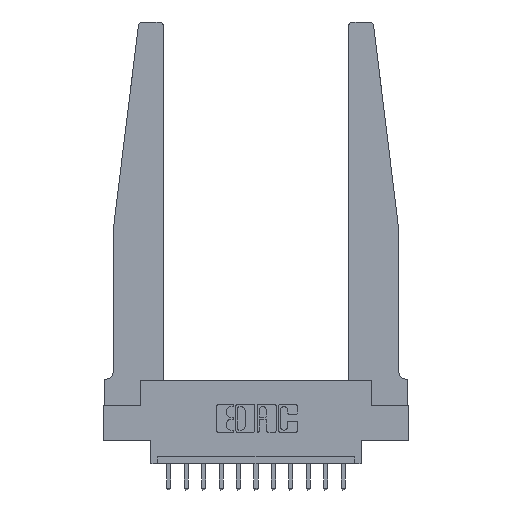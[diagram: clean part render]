
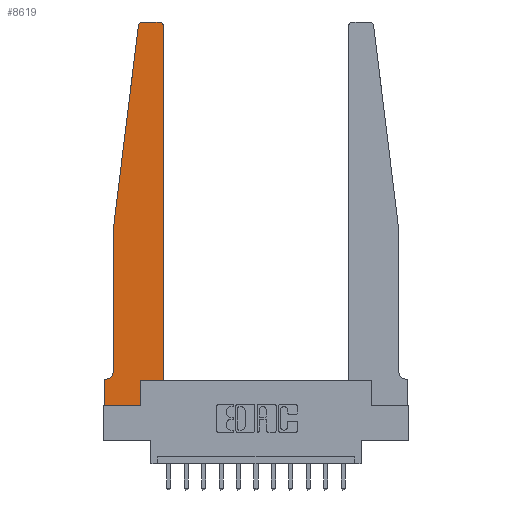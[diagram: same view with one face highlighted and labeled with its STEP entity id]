
A CAD part, top view. The second image highlights one B-rep face of the part: STEP entity #8619.
In plain terms, the highlighted planar face has unit normal (0, 0, 1).
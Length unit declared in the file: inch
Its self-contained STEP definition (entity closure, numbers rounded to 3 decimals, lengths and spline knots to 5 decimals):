
#28 = EDGE_CURVE ( 'NONE', #14382, #12071, #12122, .T. ) ;
#48 = CARTESIAN_POINT ( 'NONE',  ( 0.27653, 2.72, 0.37 ) ) ;
#54 = CARTESIAN_POINT ( 'NONE',  ( 0.27653, 2.75, 0.37 ) ) ;
#394 = CARTESIAN_POINT ( 'NONE',  ( 0.425, 0.18, 0.37 ) ) ;
#505 = LINE ( 'NONE', #9838, #10966 ) ;
#746 = EDGE_CURVE ( 'NONE', #7566, #3787, #5957, .T. ) ;
#974 = CIRCLE ( 'NONE', #13936, 0.03 ) ;
#1080 = ORIENTED_EDGE ( 'NONE', *, *, #1989, .T. ) ;
#1098 = VERTEX_POINT ( 'NONE', #54 ) ;
#1146 = EDGE_CURVE ( 'NONE', #8508, #3906, #505, .T. ) ;
#1158 = LINE ( 'NONE', #11549, #9506 ) ;
#1288 = DIRECTION ( 'NONE',  ( 0., 0., 1. ) ) ;
#1580 = CARTESIAN_POINT ( 'NONE',  ( 0., 0.1875, 0.37 ) ) ;
#1983 = CARTESIAN_POINT ( 'NONE',  ( 0., 0., 0.37 ) ) ;
#1989 = EDGE_CURVE ( 'NONE', #6457, #1098, #10658, .T. ) ;
#2303 = DIRECTION ( 'NONE',  ( 0., 0., -1. ) ) ;
#2360 = EDGE_CURVE ( 'NONE', #13261, #15558, #4961, .T. ) ;
#2396 = VECTOR ( 'NONE', #4013, 39.37008 ) ;
#2405 = DIRECTION ( 'NONE',  ( -1., 0., 0. ) ) ;
#2742 = DIRECTION ( 'NONE',  ( 0., 1., 0. ) ) ;
#2877 = EDGE_CURVE ( 'NONE', #1098, #14382, #974, .T. ) ;
#2994 = CARTESIAN_POINT ( 'NONE',  ( 0.065, 1.25, 0.37 ) ) ;
#3413 = CIRCLE ( 'NONE', #8159, 0.05 ) ;
#3787 = VERTEX_POINT ( 'NONE', #10122 ) ;
#3796 = DIRECTION ( 'NONE',  ( 1., 0., 0. ) ) ;
#3899 = CARTESIAN_POINT ( 'NONE',  ( 0., 0.1875, 0.37 ) ) ;
#3906 = VERTEX_POINT ( 'NONE', #1580 ) ;
#4013 = DIRECTION ( 'NONE',  ( -0.122, -0.992, 0. ) ) ;
#4871 = ORIENTED_EDGE ( 'NONE', *, *, #2877, .T. ) ;
#4961 = LINE ( 'NONE', #394, #12158 ) ;
#5356 = DIRECTION ( 'NONE',  ( 1., 0., 0. ) ) ;
#5385 = CARTESIAN_POINT ( 'NONE',  ( 0., 0., 0.37 ) ) ;
#5846 = CARTESIAN_POINT ( 'NONE',  ( 0.2605, 0., 0.37 ) ) ;
#5957 = LINE ( 'NONE', #9112, #7497 ) ;
#6034 = CARTESIAN_POINT ( 'NONE',  ( 0.065, 1.25, 0.37 ) ) ;
#6059 = CARTESIAN_POINT ( 'NONE',  ( 0.065, 0.2375, 0.37 ) ) ;
#6457 = VERTEX_POINT ( 'NONE', #13063 ) ;
#6497 = DIRECTION ( 'NONE',  ( 1., 0., 0. ) ) ;
#6734 = EDGE_CURVE ( 'NONE', #3787, #13261, #1158, .T. ) ;
#7161 = EDGE_CURVE ( 'NONE', #3906, #9152, #12614, .T. ) ;
#7271 = VERTEX_POINT ( 'NONE', #6059 ) ;
#7497 = VECTOR ( 'NONE', #15308, 39.37008 ) ;
#7566 = VERTEX_POINT ( 'NONE', #5846 ) ;
#7696 = ORIENTED_EDGE ( 'NONE', *, *, #6734, .T. ) ;
#7759 = ORIENTED_EDGE ( 'NONE', *, *, #1146, .T. ) ;
#7770 = DIRECTION ( 'NONE',  ( 1., 0., 0. ) ) ;
#8121 = ORIENTED_EDGE ( 'NONE', *, *, #15650, .T. ) ;
#8159 = AXIS2_PLACEMENT_3D ( 'NONE', #12286, #2303, #2405 ) ;
#8188 = CARTESIAN_POINT ( 'NONE',  ( 0.24675, 2.72367, 0.37 ) ) ;
#8312 = DIRECTION ( 'NONE',  ( 0., -1., 0. ) ) ;
#8508 = VERTEX_POINT ( 'NONE', #12459 ) ;
#8619 = ADVANCED_FACE ( 'NONE', ( #10020 ), #11304, .T. ) ;
#8872 = VECTOR ( 'NONE', #6497, 39.37008 ) ;
#9112 = CARTESIAN_POINT ( 'NONE',  ( 0.2605, 0.18, 0.37 ) ) ;
#9152 = VERTEX_POINT ( 'NONE', #14623 ) ;
#9506 = VECTOR ( 'NONE', #7770, 39.37008 ) ;
#9586 = EDGE_CURVE ( 'NONE', #15558, #6457, #14068, .T. ) ;
#9811 = DIRECTION ( 'NONE',  ( -1., 0., 0. ) ) ;
#9838 = CARTESIAN_POINT ( 'NONE',  ( 0.065, 0.1875, 0.37 ) ) ;
#10020 = FACE_OUTER_BOUND ( 'NONE', #10627, .T. ) ;
#10122 = CARTESIAN_POINT ( 'NONE',  ( 0.2605, 0.18, 0.37 ) ) ;
#10144 = CARTESIAN_POINT ( 'NONE',  ( 0.395, 2.72, 0.37 ) ) ;
#10512 = CARTESIAN_POINT ( 'NONE',  ( 0.425, 2.72, 0.37 ) ) ;
#10627 = EDGE_LOOP ( 'NONE', ( #1080, #4871, #12989, #8121, #11871, #7759, #12220, #13383, #12340, #7696, #14231, #16010 ) ) ;
#10658 = LINE ( 'NONE', #13601, #15856 ) ;
#10966 = VECTOR ( 'NONE', #11104, 39.37008 ) ;
#11040 = EDGE_CURVE ( 'NONE', #7271, #8508, #3413, .T. ) ;
#11104 = DIRECTION ( 'NONE',  ( -1., 0., 0. ) ) ;
#11304 = PLANE ( 'NONE',  #14538 ) ;
#11547 = DIRECTION ( 'NONE',  ( 0., 0., 1. ) ) ;
#11549 = CARTESIAN_POINT ( 'NONE',  ( 0.425, 0.18, 0.37 ) ) ;
#11623 = LINE ( 'NONE', #5385, #8872 ) ;
#11871 = ORIENTED_EDGE ( 'NONE', *, *, #11040, .T. ) ;
#12071 = VERTEX_POINT ( 'NONE', #6034 ) ;
#12122 = LINE ( 'NONE', #2994, #2396 ) ;
#12158 = VECTOR ( 'NONE', #2742, 39.37008 ) ;
#12220 = ORIENTED_EDGE ( 'NONE', *, *, #7161, .T. ) ;
#12286 = CARTESIAN_POINT ( 'NONE',  ( 0.015, 0.2375, 0.37 ) ) ;
#12340 = ORIENTED_EDGE ( 'NONE', *, *, #746, .T. ) ;
#12459 = CARTESIAN_POINT ( 'NONE',  ( 0.015, 0.1875, 0.37 ) ) ;
#12614 = LINE ( 'NONE', #1983, #12801 ) ;
#12801 = VECTOR ( 'NONE', #14298, 39.37008 ) ;
#12989 = ORIENTED_EDGE ( 'NONE', *, *, #28, .T. ) ;
#13063 = CARTESIAN_POINT ( 'NONE',  ( 0.395, 2.75, 0.37 ) ) ;
#13261 = VERTEX_POINT ( 'NONE', #15117 ) ;
#13383 = ORIENTED_EDGE ( 'NONE', *, *, #13686, .T. ) ;
#13412 = DIRECTION ( 'NONE',  ( 1., 0., 0. ) ) ;
#13465 = VECTOR ( 'NONE', #8312, 39.37008 ) ;
#13601 = CARTESIAN_POINT ( 'NONE',  ( 0.25, 2.75, 0.37 ) ) ;
#13686 = EDGE_CURVE ( 'NONE', #9152, #7566, #11623, .T. ) ;
#13835 = LINE ( 'NONE', #14472, #13465 ) ;
#13936 = AXIS2_PLACEMENT_3D ( 'NONE', #48, #1288, #3796 ) ;
#14068 = CIRCLE ( 'NONE', #15786, 0.03 ) ;
#14231 = ORIENTED_EDGE ( 'NONE', *, *, #2360, .T. ) ;
#14298 = DIRECTION ( 'NONE',  ( 0., -1., 0. ) ) ;
#14382 = VERTEX_POINT ( 'NONE', #8188 ) ;
#14472 = CARTESIAN_POINT ( 'NONE',  ( 0.065, 1.25, 0.37 ) ) ;
#14538 = AXIS2_PLACEMENT_3D ( 'NONE', #3899, #11547, #5356 ) ;
#14623 = CARTESIAN_POINT ( 'NONE',  ( 0., 0., 0.37 ) ) ;
#14804 = DIRECTION ( 'NONE',  ( 0., 0., 1. ) ) ;
#15117 = CARTESIAN_POINT ( 'NONE',  ( 0.425, 0.18, 0.37 ) ) ;
#15308 = DIRECTION ( 'NONE',  ( 0., 1., 0. ) ) ;
#15558 = VERTEX_POINT ( 'NONE', #10512 ) ;
#15650 = EDGE_CURVE ( 'NONE', #12071, #7271, #13835, .T. ) ;
#15786 = AXIS2_PLACEMENT_3D ( 'NONE', #10144, #14804, #13412 ) ;
#15856 = VECTOR ( 'NONE', #9811, 39.37008 ) ;
#16010 = ORIENTED_EDGE ( 'NONE', *, *, #9586, .T. ) ;
